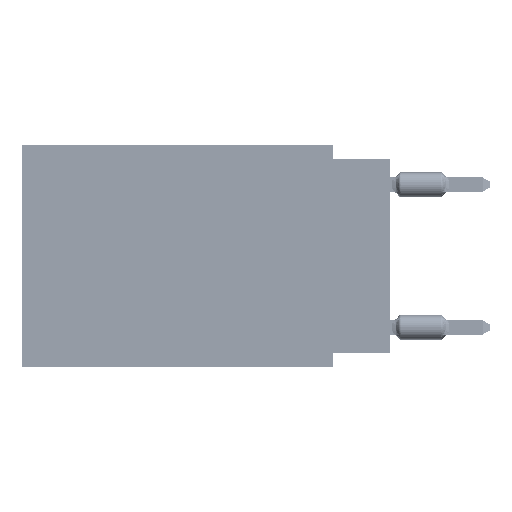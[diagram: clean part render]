
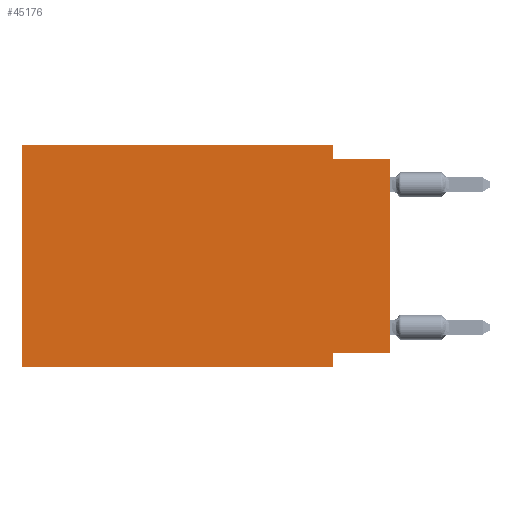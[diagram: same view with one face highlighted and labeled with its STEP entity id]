
A CAD part, left-side view. The second image highlights one B-rep face of the part: STEP entity #45176.
In plain terms, the highlighted planar face has unit normal (-1, 0, 0).
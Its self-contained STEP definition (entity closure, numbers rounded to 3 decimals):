
#824 = LINE ( 'NONE', #68425, #66148 ) ;
#1173 = DIRECTION ( 'NONE',  ( 0., -1., 0. ) ) ;
#2453 = CARTESIAN_POINT ( 'NONE',  ( 0., 2.54, -9.906 ) ) ;
#2814 = LINE ( 'NONE', #2453, #69001 ) ;
#4278 = VERTEX_POINT ( 'NONE', #22368 ) ;
#6499 = VECTOR ( 'NONE', #70658, 1000. ) ;
#9027 = CARTESIAN_POINT ( 'NONE',  ( 0., 2.54, -9.906 ) ) ;
#9216 = ORIENTED_EDGE ( 'NONE', *, *, #56691, .F. ) ;
#11454 = CARTESIAN_POINT ( 'NONE',  ( 0., 16.383, 0. ) ) ;
#12493 = VECTOR ( 'NONE', #1173, 1000. ) ;
#12795 = EDGE_CURVE ( 'NONE', #52571, #45754, #34151, .T. ) ;
#14664 = ORIENTED_EDGE ( 'NONE', *, *, #23769, .F. ) ;
#15236 = CARTESIAN_POINT ( 'NONE',  ( 0., 16.383, 0. ) ) ;
#16465 = EDGE_CURVE ( 'NONE', #31398, #45754, #25005, .T. ) ;
#18255 = VECTOR ( 'NONE', #63779, 1000. ) ;
#18391 = PLANE ( 'NONE',  #59018 ) ;
#22368 = CARTESIAN_POINT ( 'NONE',  ( 0., 2.54, -9.271 ) ) ;
#23733 = CARTESIAN_POINT ( 'NONE',  ( 0., 0., 0. ) ) ;
#23769 = EDGE_CURVE ( 'NONE', #62393, #31398, #27091, .T. ) ;
#25005 = LINE ( 'NONE', #58402, #6499 ) ;
#26512 = CARTESIAN_POINT ( 'NONE',  ( 0., 2.54, 0. ) ) ;
#27091 = LINE ( 'NONE', #61603, #62910 ) ;
#29655 = CARTESIAN_POINT ( 'NONE',  ( 0., 16.383, 0. ) ) ;
#31398 = VERTEX_POINT ( 'NONE', #40138 ) ;
#32170 = ORIENTED_EDGE ( 'NONE', *, *, #71829, .F. ) ;
#33071 = VERTEX_POINT ( 'NONE', #15236 ) ;
#34151 = LINE ( 'NONE', #23733, #63099 ) ;
#34281 = VERTEX_POINT ( 'NONE', #9027 ) ;
#35589 = LINE ( 'NONE', #11454, #48851 ) ;
#37876 = DIRECTION ( 'NONE',  ( 0., 0., -1. ) ) ;
#39197 = ORIENTED_EDGE ( 'NONE', *, *, #63737, .F. ) ;
#39870 = CARTESIAN_POINT ( 'NONE',  ( 0., 0., -9.271 ) ) ;
#40138 = CARTESIAN_POINT ( 'NONE',  ( 0., 2.54, -0.635 ) ) ;
#40934 = LINE ( 'NONE', #69887, #12493 ) ;
#41137 = DIRECTION ( 'NONE',  ( 0., 0., 1. ) ) ;
#45176 = ADVANCED_FACE ( 'NONE', ( #46610 ), #18391, .F. ) ;
#45620 = LINE ( 'NONE', #29655, #18255 ) ;
#45754 = VERTEX_POINT ( 'NONE', #60972 ) ;
#46610 = FACE_OUTER_BOUND ( 'NONE', #71769, .T. ) ;
#46953 = VERTEX_POINT ( 'NONE', #72218 ) ;
#48851 = VECTOR ( 'NONE', #41137, 1000. ) ;
#51316 = ORIENTED_EDGE ( 'NONE', *, *, #60832, .F. ) ;
#51709 = DIRECTION ( 'NONE',  ( 0., 1., 0. ) ) ;
#52571 = VERTEX_POINT ( 'NONE', #39870 ) ;
#52937 = ORIENTED_EDGE ( 'NONE', *, *, #16465, .F. ) ;
#54688 = EDGE_CURVE ( 'NONE', #46953, #34281, #40934, .T. ) ;
#55714 = ORIENTED_EDGE ( 'NONE', *, *, #54688, .T. ) ;
#56691 = EDGE_CURVE ( 'NONE', #46953, #33071, #35589, .T. ) ;
#58402 = CARTESIAN_POINT ( 'NONE',  ( 0., 0., -0.635 ) ) ;
#58847 = CARTESIAN_POINT ( 'NONE',  ( 0., 16.383, 0. ) ) ;
#59018 = AXIS2_PLACEMENT_3D ( 'NONE', #58847, #69997, #63682 ) ;
#59646 = DIRECTION ( 'NONE',  ( 0., 0., -1. ) ) ;
#60832 = EDGE_CURVE ( 'NONE', #33071, #62393, #45620, .T. ) ;
#60972 = CARTESIAN_POINT ( 'NONE',  ( 0., 0., -0.635 ) ) ;
#61603 = CARTESIAN_POINT ( 'NONE',  ( 0., 2.54, 0. ) ) ;
#62393 = VERTEX_POINT ( 'NONE', #26512 ) ;
#62910 = VECTOR ( 'NONE', #37876, 1000. ) ;
#63099 = VECTOR ( 'NONE', #69372, 1000. ) ;
#63682 = DIRECTION ( 'NONE',  ( 0., 0., -1. ) ) ;
#63737 = EDGE_CURVE ( 'NONE', #52571, #4278, #824, .T. ) ;
#63779 = DIRECTION ( 'NONE',  ( 0., -1., 0. ) ) ;
#66148 = VECTOR ( 'NONE', #51709, 1000. ) ;
#68425 = CARTESIAN_POINT ( 'NONE',  ( 0., 0., -9.271 ) ) ;
#69001 = VECTOR ( 'NONE', #59646, 1000. ) ;
#69372 = DIRECTION ( 'NONE',  ( 0., 0., 1. ) ) ;
#69887 = CARTESIAN_POINT ( 'NONE',  ( 0., 16.383, -9.906 ) ) ;
#69997 = DIRECTION ( 'NONE',  ( 1., 0., 0. ) ) ;
#70604 = ORIENTED_EDGE ( 'NONE', *, *, #12795, .T. ) ;
#70658 = DIRECTION ( 'NONE',  ( 0., -1., 0. ) ) ;
#71769 = EDGE_LOOP ( 'NONE', ( #70604, #52937, #14664, #51316, #9216, #55714, #32170, #39197 ) ) ;
#71829 = EDGE_CURVE ( 'NONE', #4278, #34281, #2814, .T. ) ;
#72218 = CARTESIAN_POINT ( 'NONE',  ( 0., 16.383, -9.906 ) ) ;
